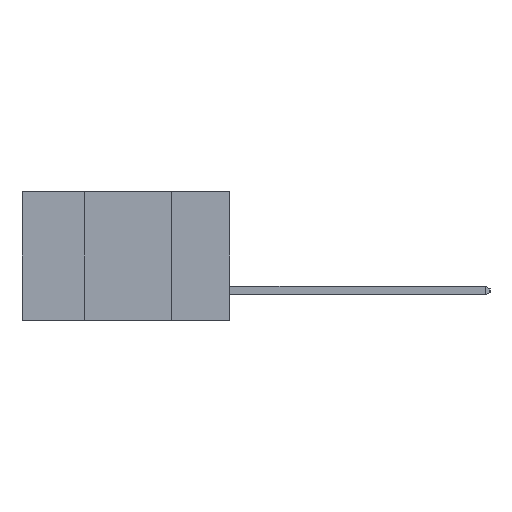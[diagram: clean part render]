
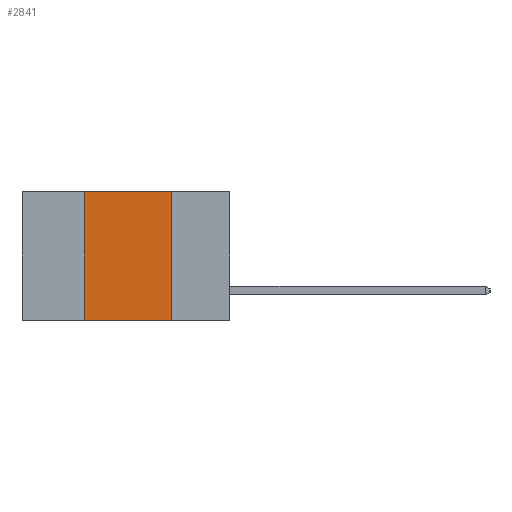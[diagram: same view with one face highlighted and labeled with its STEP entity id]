
A CAD part, left-side view. The second image highlights one B-rep face of the part: STEP entity #2841.
In plain terms, the highlighted planar face has unit normal (-1, 0, 0).
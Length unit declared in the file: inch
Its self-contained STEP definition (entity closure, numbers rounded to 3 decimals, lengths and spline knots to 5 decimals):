
#171 = ORIENTED_EDGE ( 'NONE', *, *, #3841, .F. ) ;
#376 = EDGE_CURVE ( 'NONE', #4559, #18307, #21012, .T. ) ;
#1765 = ORIENTED_EDGE ( 'NONE', *, *, #17316, .T. ) ;
#1782 = AXIS2_PLACEMENT_3D ( 'NONE', #17416, #17317, #17224 ) ;
#1831 = DIRECTION ( 'NONE',  ( 0., 0., 1. ) ) ;
#1932 = CARTESIAN_POINT ( 'NONE',  ( 0., 0.42, -0.37 ) ) ;
#2841 = ADVANCED_FACE ( 'NONE', ( #14663 ), #17514, .F. ) ;
#3315 = DIRECTION ( 'NONE',  ( 0., 0., -1. ) ) ;
#3453 = CARTESIAN_POINT ( 'NONE',  ( 0., 0.17, -0.37 ) ) ;
#3841 = EDGE_CURVE ( 'NONE', #18307, #4896, #17211, .T. ) ;
#4559 = VERTEX_POINT ( 'NONE', #20836 ) ;
#4896 = VERTEX_POINT ( 'NONE', #15063 ) ;
#5806 = ORIENTED_EDGE ( 'NONE', *, *, #14271, .F. ) ;
#6160 = VERTEX_POINT ( 'NONE', #16847 ) ;
#6381 = CARTESIAN_POINT ( 'NONE',  ( 0., 0.6, 0. ) ) ;
#9010 = VECTOR ( 'NONE', #3315, 39.37008 ) ;
#10098 = CARTESIAN_POINT ( 'NONE',  ( 0., 0.6, -0.37 ) ) ;
#10143 = DIRECTION ( 'NONE',  ( 0., -1., 0. ) ) ;
#10372 = CARTESIAN_POINT ( 'NONE',  ( 0., 0.17, 0. ) ) ;
#10669 = VECTOR ( 'NONE', #1831, 39.37008 ) ;
#11785 = EDGE_LOOP ( 'NONE', ( #171, #14076, #5806, #1765 ) ) ;
#12001 = VECTOR ( 'NONE', #19259, 39.37008 ) ;
#14076 = ORIENTED_EDGE ( 'NONE', *, *, #376, .F. ) ;
#14271 = EDGE_CURVE ( 'NONE', #6160, #4559, #19784, .T. ) ;
#14343 = VECTOR ( 'NONE', #10143, 39.37008 ) ;
#14663 = FACE_OUTER_BOUND ( 'NONE', #11785, .T. ) ;
#15063 = CARTESIAN_POINT ( 'NONE',  ( 0., 0.17, -0.37 ) ) ;
#16847 = CARTESIAN_POINT ( 'NONE',  ( 0., 0.42, -0.37 ) ) ;
#17211 = LINE ( 'NONE', #3453, #9010 ) ;
#17224 = DIRECTION ( 'NONE',  ( 0., 0., -1. ) ) ;
#17316 = EDGE_CURVE ( 'NONE', #6160, #4896, #18694, .T. ) ;
#17317 = DIRECTION ( 'NONE',  ( 1., 0., 0. ) ) ;
#17416 = CARTESIAN_POINT ( 'NONE',  ( 0., 0.6, 0. ) ) ;
#17514 = PLANE ( 'NONE',  #1782 ) ;
#18307 = VERTEX_POINT ( 'NONE', #10372 ) ;
#18694 = LINE ( 'NONE', #10098, #14343 ) ;
#19259 = DIRECTION ( 'NONE',  ( 0., -1., 0. ) ) ;
#19784 = LINE ( 'NONE', #1932, #10669 ) ;
#20836 = CARTESIAN_POINT ( 'NONE',  ( 0., 0.42, 0. ) ) ;
#21012 = LINE ( 'NONE', #6381, #12001 ) ;
